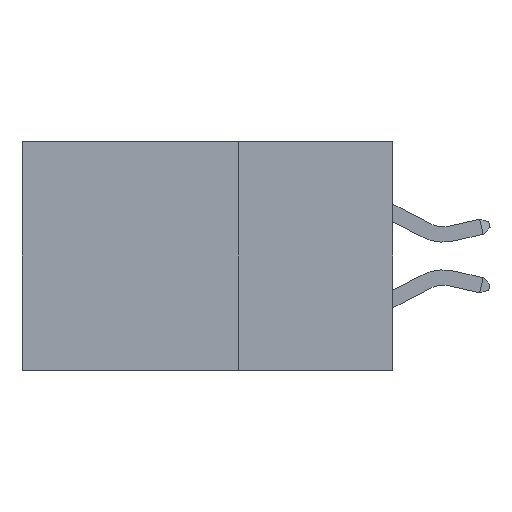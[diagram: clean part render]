
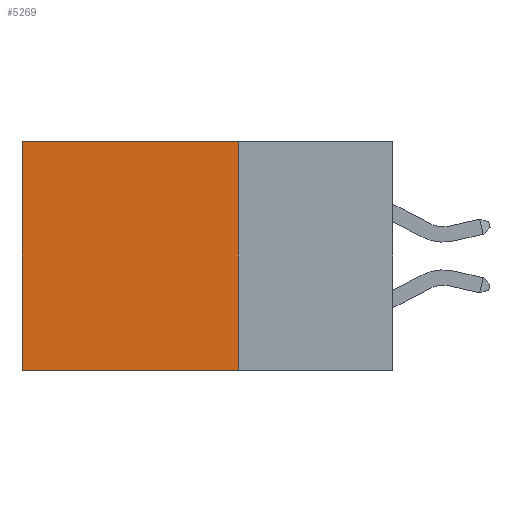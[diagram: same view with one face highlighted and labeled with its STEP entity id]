
A CAD part, left-side view. The second image highlights one B-rep face of the part: STEP entity #5269.
In plain terms, the highlighted planar face has unit normal (-1, 0, 0).
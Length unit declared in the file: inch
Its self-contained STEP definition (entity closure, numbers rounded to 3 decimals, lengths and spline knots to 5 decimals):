
#37 = VECTOR ( 'NONE', #11169, 39.37008 ) ;
#797 = FACE_OUTER_BOUND ( 'NONE', #6731, .T. ) ;
#1040 = DIRECTION ( 'NONE',  ( 0., 0., -1. ) ) ;
#1090 = VECTOR ( 'NONE', #8027, 39.37008 ) ;
#1619 = AXIS2_PLACEMENT_3D ( 'NONE', #3410, #8350, #8676 ) ;
#1971 = EDGE_CURVE ( 'NONE', #11065, #3293, #2023, .T. ) ;
#2023 = LINE ( 'NONE', #9511, #10866 ) ;
#2192 = ORIENTED_EDGE ( 'NONE', *, *, #5137, .F. ) ;
#3220 = ORIENTED_EDGE ( 'NONE', *, *, #4340, .T. ) ;
#3293 = VERTEX_POINT ( 'NONE', #4411 ) ;
#3410 = CARTESIAN_POINT ( 'NONE',  ( 0.2875, 0.25, 0. ) ) ;
#3702 = CARTESIAN_POINT ( 'NONE',  ( 0.2875, 0.25, 0. ) ) ;
#3709 = LINE ( 'NONE', #12400, #11849 ) ;
#3781 = LINE ( 'NONE', #3702, #37 ) ;
#4340 = EDGE_CURVE ( 'NONE', #11065, #8100, #3781, .T. ) ;
#4411 = CARTESIAN_POINT ( 'NONE',  ( 0.2875, 0.25, -0.37 ) ) ;
#5137 = EDGE_CURVE ( 'NONE', #3293, #10956, #14450, .T. ) ;
#5269 = ADVANCED_FACE ( 'NONE', ( #797 ), #10803, .F. ) ;
#5348 = CARTESIAN_POINT ( 'NONE',  ( 0.2875, 0.6, 0. ) ) ;
#6731 = EDGE_LOOP ( 'NONE', ( #14624, #2192, #9653, #3220 ) ) ;
#8027 = DIRECTION ( 'NONE',  ( 0., 1., 0. ) ) ;
#8100 = VERTEX_POINT ( 'NONE', #5348 ) ;
#8350 = DIRECTION ( 'NONE',  ( 1., 0., 0. ) ) ;
#8676 = DIRECTION ( 'NONE',  ( 0., 0., -1. ) ) ;
#9511 = CARTESIAN_POINT ( 'NONE',  ( 0.2875, 0.25, 0. ) ) ;
#9653 = ORIENTED_EDGE ( 'NONE', *, *, #1971, .F. ) ;
#9977 = EDGE_CURVE ( 'NONE', #8100, #10956, #3709, .T. ) ;
#10803 = PLANE ( 'NONE',  #1619 ) ;
#10866 = VECTOR ( 'NONE', #1040, 39.37008 ) ;
#10942 = DIRECTION ( 'NONE',  ( 0., 0., -1. ) ) ;
#10956 = VERTEX_POINT ( 'NONE', #14030 ) ;
#11065 = VERTEX_POINT ( 'NONE', #13870 ) ;
#11169 = DIRECTION ( 'NONE',  ( 0., 1., 0. ) ) ;
#11849 = VECTOR ( 'NONE', #10942, 39.37008 ) ;
#12400 = CARTESIAN_POINT ( 'NONE',  ( 0.2875, 0.6, 0. ) ) ;
#13245 = CARTESIAN_POINT ( 'NONE',  ( 0.2875, 0.25, -0.37 ) ) ;
#13870 = CARTESIAN_POINT ( 'NONE',  ( 0.2875, 0.25, 0. ) ) ;
#14030 = CARTESIAN_POINT ( 'NONE',  ( 0.2875, 0.6, -0.37 ) ) ;
#14450 = LINE ( 'NONE', #13245, #1090 ) ;
#14624 = ORIENTED_EDGE ( 'NONE', *, *, #9977, .T. ) ;
